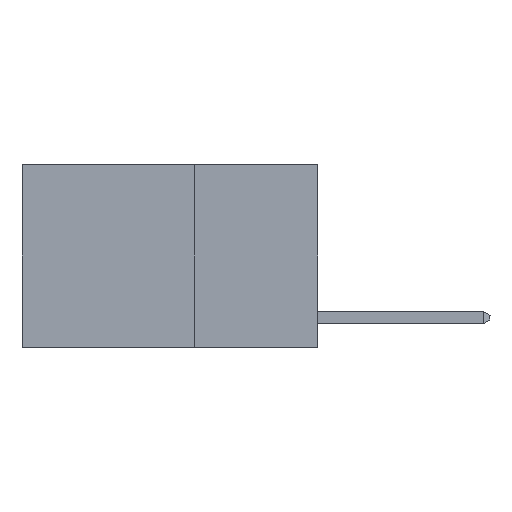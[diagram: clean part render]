
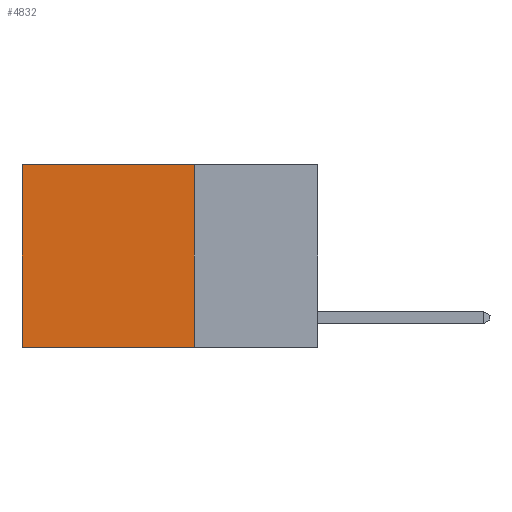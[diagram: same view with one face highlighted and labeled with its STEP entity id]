
A CAD part, left-side view. The second image highlights one B-rep face of the part: STEP entity #4832.
In plain terms, the highlighted planar face has unit normal (-1, 0, 0).
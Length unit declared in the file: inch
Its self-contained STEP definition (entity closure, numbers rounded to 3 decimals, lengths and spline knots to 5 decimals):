
#329 = EDGE_CURVE ( 'NONE', #3681, #11518, #9417, .T. ) ;
#930 = VECTOR ( 'NONE', #5291, 39.37008 ) ;
#1229 = VECTOR ( 'NONE', #9314, 39.37008 ) ;
#2004 = EDGE_CURVE ( 'NONE', #8642, #11518, #10668, .T. ) ;
#2262 = PLANE ( 'NONE',  #5555 ) ;
#2297 = FACE_OUTER_BOUND ( 'NONE', #3792, .T. ) ;
#2750 = EDGE_CURVE ( 'NONE', #7573, #8642, #5866, .T. ) ;
#2865 = EDGE_CURVE ( 'NONE', #7573, #3681, #3374, .T. ) ;
#3374 = LINE ( 'NONE', #10039, #930 ) ;
#3506 = CARTESIAN_POINT ( 'NONE',  ( 0.2625, 0.6, 0. ) ) ;
#3571 = CARTESIAN_POINT ( 'NONE',  ( 0.2625, 0.6, 0. ) ) ;
#3681 = VERTEX_POINT ( 'NONE', #6228 ) ;
#3792 = EDGE_LOOP ( 'NONE', ( #5733, #7682, #6305, #8404 ) ) ;
#4832 = ADVANCED_FACE ( 'NONE', ( #2297 ), #2262, .F. ) ;
#5039 = CARTESIAN_POINT ( 'NONE',  ( 0.2625, 0.25, 0. ) ) ;
#5291 = DIRECTION ( 'NONE',  ( 0., 0., -1. ) ) ;
#5555 = AXIS2_PLACEMENT_3D ( 'NONE', #5039, #8780, #9589 ) ;
#5733 = ORIENTED_EDGE ( 'NONE', *, *, #2004, .T. ) ;
#5866 = LINE ( 'NONE', #6570, #1229 ) ;
#6128 = CARTESIAN_POINT ( 'NONE',  ( 0.2625, 0.6, -0.37 ) ) ;
#6225 = DIRECTION ( 'NONE',  ( 0., 0., -1. ) ) ;
#6228 = CARTESIAN_POINT ( 'NONE',  ( 0.2625, 0.25, -0.37 ) ) ;
#6305 = ORIENTED_EDGE ( 'NONE', *, *, #2865, .F. ) ;
#6570 = CARTESIAN_POINT ( 'NONE',  ( 0.2625, 0.25, 0. ) ) ;
#7543 = VECTOR ( 'NONE', #9900, 39.37008 ) ;
#7573 = VERTEX_POINT ( 'NONE', #10911 ) ;
#7682 = ORIENTED_EDGE ( 'NONE', *, *, #329, .F. ) ;
#8232 = VECTOR ( 'NONE', #6225, 39.37008 ) ;
#8241 = CARTESIAN_POINT ( 'NONE',  ( 0.2625, 0.25, -0.37 ) ) ;
#8404 = ORIENTED_EDGE ( 'NONE', *, *, #2750, .T. ) ;
#8642 = VERTEX_POINT ( 'NONE', #3506 ) ;
#8780 = DIRECTION ( 'NONE',  ( 1., 0., 0. ) ) ;
#9314 = DIRECTION ( 'NONE',  ( 0., 1., 0. ) ) ;
#9417 = LINE ( 'NONE', #8241, #7543 ) ;
#9589 = DIRECTION ( 'NONE',  ( 0., 0., -1. ) ) ;
#9900 = DIRECTION ( 'NONE',  ( 0., 1., 0. ) ) ;
#10039 = CARTESIAN_POINT ( 'NONE',  ( 0.2625, 0.25, 0. ) ) ;
#10668 = LINE ( 'NONE', #3571, #8232 ) ;
#10911 = CARTESIAN_POINT ( 'NONE',  ( 0.2625, 0.25, 0. ) ) ;
#11518 = VERTEX_POINT ( 'NONE', #6128 ) ;
